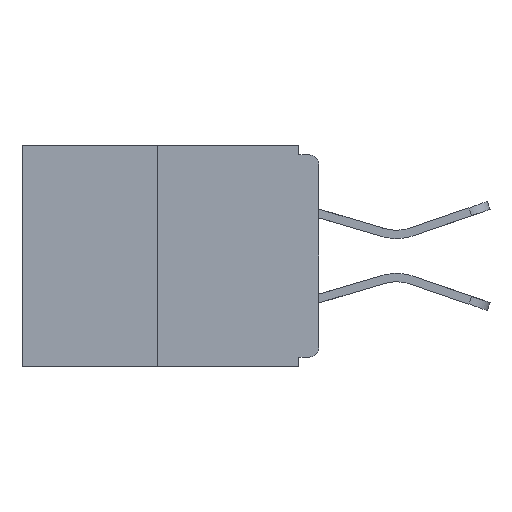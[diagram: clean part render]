
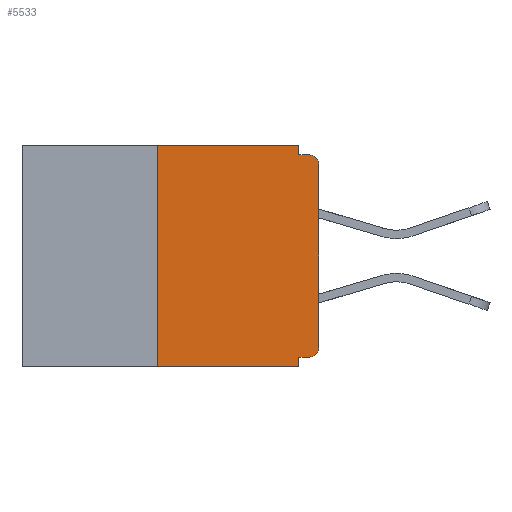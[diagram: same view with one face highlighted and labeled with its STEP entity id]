
A CAD part, left-side view. The second image highlights one B-rep face of the part: STEP entity #5533.
In plain terms, the highlighted planar face has unit normal (-1, 0, 0).
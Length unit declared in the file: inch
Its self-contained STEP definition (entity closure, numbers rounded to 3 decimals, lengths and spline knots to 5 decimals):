
#275 = LINE ( 'NONE', #16748, #2362 ) ;
#297 = EDGE_CURVE ( 'NONE', #2156, #7934, #9990, .T. ) ;
#386 = CIRCLE ( 'NONE', #3234, 0.015 ) ;
#515 = EDGE_CURVE ( 'NONE', #14570, #2156, #6677, .T. ) ;
#1059 = DIRECTION ( 'NONE',  ( 0., 0., -1. ) ) ;
#1163 = CARTESIAN_POINT ( 'NONE',  ( 0., 0.031, -0.343 ) ) ;
#1217 = CARTESIAN_POINT ( 'NONE',  ( 0., 0.015, -0.313 ) ) ;
#1406 = CARTESIAN_POINT ( 'NONE',  ( 0., 0.015, -0.03 ) ) ;
#1423 = CARTESIAN_POINT ( 'NONE',  ( 0., 0.25, -0.343 ) ) ;
#1450 = CARTESIAN_POINT ( 'NONE',  ( 0., 0.015, -0.015 ) ) ;
#1642 = ORIENTED_EDGE ( 'NONE', *, *, #8693, .T. ) ;
#2156 = VERTEX_POINT ( 'NONE', #12908 ) ;
#2173 = AXIS2_PLACEMENT_3D ( 'NONE', #1406, #8037, #1059 ) ;
#2280 = LINE ( 'NONE', #8104, #15490 ) ;
#2362 = VECTOR ( 'NONE', #12612, 39.37008 ) ;
#2434 = ORIENTED_EDGE ( 'NONE', *, *, #15578, .T. ) ;
#2476 = CARTESIAN_POINT ( 'NONE',  ( 0., 0., -0.313 ) ) ;
#2660 = CARTESIAN_POINT ( 'NONE',  ( 0., 0., -0.03 ) ) ;
#2859 = CARTESIAN_POINT ( 'NONE',  ( 0., 0.031, -0.343 ) ) ;
#3234 = AXIS2_PLACEMENT_3D ( 'NONE', #1217, #17507, #16155 ) ;
#3293 = LINE ( 'NONE', #11422, #16478 ) ;
#4014 = VERTEX_POINT ( 'NONE', #6193 ) ;
#4095 = EDGE_CURVE ( 'NONE', #5541, #8608, #11631, .T. ) ;
#5368 = DIRECTION ( 'NONE',  ( 1., 0., 0. ) ) ;
#5533 = ADVANCED_FACE ( 'NONE', ( #10645 ), #7978, .F. ) ;
#5538 = ORIENTED_EDGE ( 'NONE', *, *, #297, .F. ) ;
#5541 = VERTEX_POINT ( 'NONE', #1423 ) ;
#5742 = CARTESIAN_POINT ( 'NONE',  ( 0., 0.031, 0. ) ) ;
#5974 = ORIENTED_EDGE ( 'NONE', *, *, #8199, .F. ) ;
#6193 = CARTESIAN_POINT ( 'NONE',  ( 0., 0.015, -0.328 ) ) ;
#6291 = ORIENTED_EDGE ( 'NONE', *, *, #6545, .F. ) ;
#6545 = EDGE_CURVE ( 'NONE', #8608, #14570, #2280, .T. ) ;
#6677 = LINE ( 'NONE', #5742, #10470 ) ;
#6756 = CIRCLE ( 'NONE', #2173, 0.015 ) ;
#6814 = DIRECTION ( 'NONE',  ( 0., 0., -1. ) ) ;
#7934 = VERTEX_POINT ( 'NONE', #1450 ) ;
#7978 = PLANE ( 'NONE',  #13224 ) ;
#8037 = DIRECTION ( 'NONE',  ( -1., 0., 0. ) ) ;
#8104 = CARTESIAN_POINT ( 'NONE',  ( 0., 0.46, 0. ) ) ;
#8199 = EDGE_CURVE ( 'NONE', #17067, #8229, #8330, .T. ) ;
#8229 = VERTEX_POINT ( 'NONE', #2859 ) ;
#8330 = LINE ( 'NONE', #1163, #14138 ) ;
#8355 = CARTESIAN_POINT ( 'NONE',  ( 0., 0., 0. ) ) ;
#8608 = VERTEX_POINT ( 'NONE', #12867 ) ;
#8693 = EDGE_CURVE ( 'NONE', #8707, #7934, #6756, .T. ) ;
#8707 = VERTEX_POINT ( 'NONE', #2660 ) ;
#8813 = CARTESIAN_POINT ( 'NONE',  ( 0., 0.031, -0.328 ) ) ;
#9103 = DIRECTION ( 'NONE',  ( 0., -1., 0. ) ) ;
#9225 = ORIENTED_EDGE ( 'NONE', *, *, #10112, .T. ) ;
#9395 = ORIENTED_EDGE ( 'NONE', *, *, #4095, .F. ) ;
#9465 = ORIENTED_EDGE ( 'NONE', *, *, #515, .F. ) ;
#9695 = LINE ( 'NONE', #8355, #14699 ) ;
#9990 = LINE ( 'NONE', #14008, #14755 ) ;
#10002 = DIRECTION ( 'NONE',  ( 0., -1., 0. ) ) ;
#10112 = EDGE_CURVE ( 'NONE', #5541, #8229, #3293, .T. ) ;
#10363 = VERTEX_POINT ( 'NONE', #2476 ) ;
#10470 = VECTOR ( 'NONE', #14799, 39.37008 ) ;
#10645 = FACE_OUTER_BOUND ( 'NONE', #16845, .T. ) ;
#11129 = VECTOR ( 'NONE', #15921, 39.37008 ) ;
#11422 = CARTESIAN_POINT ( 'NONE',  ( 0., 0.46, -0.343 ) ) ;
#11631 = LINE ( 'NONE', #17101, #11129 ) ;
#12612 = DIRECTION ( 'NONE',  ( 0., 1., 0. ) ) ;
#12675 = DIRECTION ( 'NONE',  ( 0., -1., 0. ) ) ;
#12867 = CARTESIAN_POINT ( 'NONE',  ( 0., 0.25, 0. ) ) ;
#12908 = CARTESIAN_POINT ( 'NONE',  ( 0., 0.031, -0.015 ) ) ;
#13224 = AXIS2_PLACEMENT_3D ( 'NONE', #17638, #5368, #6814 ) ;
#13327 = ORIENTED_EDGE ( 'NONE', *, *, #16889, .T. ) ;
#13500 = ORIENTED_EDGE ( 'NONE', *, *, #14731, .F. ) ;
#14008 = CARTESIAN_POINT ( 'NONE',  ( 0., 0., -0.015 ) ) ;
#14138 = VECTOR ( 'NONE', #14845, 39.37008 ) ;
#14570 = VERTEX_POINT ( 'NONE', #15851 ) ;
#14699 = VECTOR ( 'NONE', #17666, 39.37008 ) ;
#14731 = EDGE_CURVE ( 'NONE', #4014, #17067, #275, .T. ) ;
#14755 = VECTOR ( 'NONE', #12675, 39.37008 ) ;
#14799 = DIRECTION ( 'NONE',  ( 0., 0., -1. ) ) ;
#14845 = DIRECTION ( 'NONE',  ( 0., 0., -1. ) ) ;
#15490 = VECTOR ( 'NONE', #9103, 39.37008 ) ;
#15578 = EDGE_CURVE ( 'NONE', #4014, #10363, #386, .T. ) ;
#15851 = CARTESIAN_POINT ( 'NONE',  ( 0., 0.031, 0. ) ) ;
#15921 = DIRECTION ( 'NONE',  ( 0., 0., 1. ) ) ;
#16155 = DIRECTION ( 'NONE',  ( 0., 0., -1. ) ) ;
#16478 = VECTOR ( 'NONE', #10002, 39.37008 ) ;
#16748 = CARTESIAN_POINT ( 'NONE',  ( 0., 0., -0.328 ) ) ;
#16845 = EDGE_LOOP ( 'NONE', ( #6291, #9395, #9225, #5974, #13500, #2434, #13327, #1642, #5538, #9465 ) ) ;
#16889 = EDGE_CURVE ( 'NONE', #10363, #8707, #9695, .T. ) ;
#17067 = VERTEX_POINT ( 'NONE', #8813 ) ;
#17101 = CARTESIAN_POINT ( 'NONE',  ( 0., 0.25, 0. ) ) ;
#17507 = DIRECTION ( 'NONE',  ( -1., 0., 0. ) ) ;
#17638 = CARTESIAN_POINT ( 'NONE',  ( 0., 0.46, 0. ) ) ;
#17666 = DIRECTION ( 'NONE',  ( 0., 0., 1. ) ) ;
